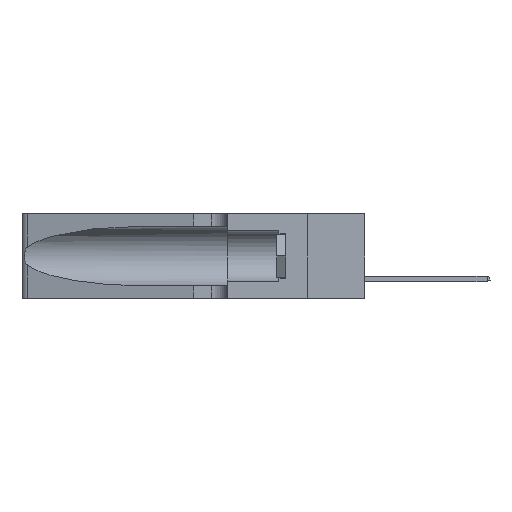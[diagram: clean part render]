
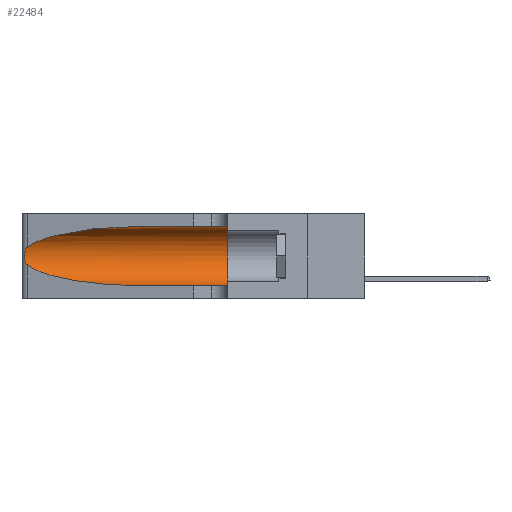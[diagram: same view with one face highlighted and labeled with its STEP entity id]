
A CAD part, left-side view. The second image highlights one B-rep face of the part: STEP entity #22484.
In plain terms, the highlighted cylindrical face has radius 3.308 mm (diameter 6.617 mm), a partial arc.
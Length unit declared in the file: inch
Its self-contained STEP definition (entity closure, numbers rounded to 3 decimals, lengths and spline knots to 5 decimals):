
#116 = DIRECTION ( 'NONE',  ( 0., -1., 0. ) ) ;
#454 = CARTESIAN_POINT ( 'NONE',  ( 0.18966, 0.96281, 0.05475 ) ) ;
#629 = CARTESIAN_POINT ( 'NONE',  ( 0.25787, 1.23484, 0.2124 ) ) ;
#763 = CARTESIAN_POINT ( 'NONE',  ( 0.25487, 1.22718, 0.14631 ) ) ;
#894 = CARTESIAN_POINT ( 'NONE',  ( 0.25555, 1.22994, 0.2215 ) ) ;
#1622 = EDGE_CURVE ( 'NONE', #23944, #12899, #24388, .T. ) ;
#1843 =( BOUNDED_CURVE ( )  B_SPLINE_CURVE ( 3, ( #36848, #27857, #454, #36561 ),
 .UNSPECIFIED., .F., .F. ) 
 B_SPLINE_CURVE_WITH_KNOTS ( ( 4, 4 ),
 ( 3.44316, 4.71239 ),
 .UNSPECIFIED. ) 
 CURVE ( )  GEOMETRIC_REPRESENTATION_ITEM ( )  RATIONAL_B_SPLINE_CURVE ( ( 1., 0.87, 0.87, 1. ) ) 
 REPRESENTATION_ITEM ( '' )  );
#3051 = LINE ( 'NONE', #29925, #14164 ) ;
#3424 = CARTESIAN_POINT ( 'NONE',  ( 0.26075, 1.23896, 0.19203 ) ) ;
#3725 = AXIS2_PLACEMENT_3D ( 'NONE', #30386, #30135, #12886 ) ;
#4051 = CARTESIAN_POINT ( 'NONE',  ( 0.1305, 0.35, 0.185 ) ) ;
#4172 = EDGE_CURVE ( 'NONE', #12899, #24948, #28204, .T. ) ;
#4389 = CARTESIAN_POINT ( 'NONE',  ( 0.25487, 1.22718, 0.14631 ) ) ;
#4609 = ORIENTED_EDGE ( 'NONE', *, *, #21694, .T. ) ;
#6536 = CARTESIAN_POINT ( 'NONE',  ( 0.1305, 0.35, 0.31525 ) ) ;
#8835 = CARTESIAN_POINT ( 'NONE',  ( 0.25856, 1.23593, 0.16098 ) ) ;
#10530 = CARTESIAN_POINT ( 'NONE',  ( 0.2373, 1.15595, 0.28018 ) ) ;
#11841 = ORIENTED_EDGE ( 'NONE', *, *, #25390, .T. ) ;
#12189 = CARTESIAN_POINT ( 'NONE',  ( 0.26018, 1.23835, 0.19895 ) ) ;
#12886 = DIRECTION ( 'NONE',  ( 0., 0., -1. ) ) ;
#12899 = VERTEX_POINT ( 'NONE', #6536 ) ;
#14164 = VECTOR ( 'NONE', #32774, 39.37008 ) ;
#15086 = CARTESIAN_POINT ( 'NONE',  ( 0.25789, 1.23486, 0.15765 ) ) ;
#15476 = DIRECTION ( 'NONE',  ( 0., 0., 1. ) ) ;
#16422 = CARTESIAN_POINT ( 'NONE',  ( 0.1305, 0.72297, 0.31525 ) ) ;
#16817 = VECTOR ( 'NONE', #116, 39.37008 ) ;
#16911 = AXIS2_PLACEMENT_3D ( 'NONE', #4051, #18142, #15476 ) ;
#16933 = EDGE_CURVE ( 'NONE', #23944, #20963, #36050, .T. ) ;
#17014 = CARTESIAN_POINT ( 'NONE',  ( 0.25487, 1.22718, 0.22369 ) ) ;
#17387 = EDGE_LOOP ( 'NONE', ( #27782, #11841, #26075, #4609, #18906, #19441 ) ) ;
#17864 = CARTESIAN_POINT ( 'NONE',  ( 0.25854, 1.2359, 0.20912 ) ) ;
#18142 = DIRECTION ( 'NONE',  ( 0., 1., 0. ) ) ;
#18906 = ORIENTED_EDGE ( 'NONE', *, *, #4172, .F. ) ;
#19441 = ORIENTED_EDGE ( 'NONE', *, *, #1622, .F. ) ;
#19479 = CARTESIAN_POINT ( 'NONE',  ( 0.25487, 1.22718, 0.22369 ) ) ;
#20963 = VERTEX_POINT ( 'NONE', #17014 ) ;
#21694 = EDGE_CURVE ( 'NONE', #27666, #24948, #3051, .T. ) ;
#21735 = VERTEX_POINT ( 'NONE', #4389 ) ;
#22058 = EDGE_CURVE ( 'NONE', #21735, #27666, #1843, .T. ) ;
#22484 = ADVANCED_FACE ( 'NONE', ( #23024 ), #25292, .F. ) ;
#22917 = CARTESIAN_POINT ( 'NONE',  ( 0.1305, 1.61858, 0.31525 ) ) ;
#23024 = FACE_OUTER_BOUND ( 'NONE', #17387, .T. ) ;
#23563 = CARTESIAN_POINT ( 'NONE',  ( 0.26017, 1.23833, 0.17102 ) ) ;
#23944 = VERTEX_POINT ( 'NONE', #32607 ) ;
#24388 = LINE ( 'NONE', #22917, #16817 ) ;
#24948 = VERTEX_POINT ( 'NONE', #26966 ) ;
#25292 = CYLINDRICAL_SURFACE ( 'NONE', #3725, 0.13025 ) ;
#25390 = EDGE_CURVE ( 'NONE', #20963, #21735, #28325, .T. ) ;
#26075 = ORIENTED_EDGE ( 'NONE', *, *, #22058, .T. ) ;
#26295 = CARTESIAN_POINT ( 'NONE',  ( 0.1305, 0.72297, 0.05475 ) ) ;
#26966 = CARTESIAN_POINT ( 'NONE',  ( 0.1305, 0.35, 0.05475 ) ) ;
#27666 = VERTEX_POINT ( 'NONE', #26295 ) ;
#27782 = ORIENTED_EDGE ( 'NONE', *, *, #16933, .T. ) ;
#27857 = CARTESIAN_POINT ( 'NONE',  ( 0.2373, 1.15595, 0.08982 ) ) ;
#28204 = CIRCLE ( 'NONE', #16911, 0.13025 ) ;
#28325 = B_SPLINE_CURVE_WITH_KNOTS ( 'NONE', 3,
 ( #32021, #894, #32163, #629, #17864, #12189, #3424, #29309, #23563, #8835, #15086, #29056, #28942, #763 ),
 .UNSPECIFIED., .F., .F.,
 ( 4, 2, 2, 2, 2, 2, 4 ),
 ( 0., 0.00027, 0.00053, 0.00107, 0.0016, 0.00187, 0.00214 ),
 .UNSPECIFIED. ) ;
#28942 = CARTESIAN_POINT ( 'NONE',  ( 0.25555, 1.22993, 0.14849 ) ) ;
#29056 = CARTESIAN_POINT ( 'NONE',  ( 0.25639, 1.23186, 0.15144 ) ) ;
#29309 = CARTESIAN_POINT ( 'NONE',  ( 0.26075, 1.23896, 0.178 ) ) ;
#29925 = CARTESIAN_POINT ( 'NONE',  ( 0.1305, 1.61858, 0.05475 ) ) ;
#30135 = DIRECTION ( 'NONE',  ( 0., -1., 0. ) ) ;
#30386 = CARTESIAN_POINT ( 'NONE',  ( 0.1305, 1.61858, 0.185 ) ) ;
#32021 = CARTESIAN_POINT ( 'NONE',  ( 0.25487, 1.22718, 0.22369 ) ) ;
#32163 = CARTESIAN_POINT ( 'NONE',  ( 0.25639, 1.23184, 0.21858 ) ) ;
#32607 = CARTESIAN_POINT ( 'NONE',  ( 0.1305, 0.72297, 0.31525 ) ) ;
#32774 = DIRECTION ( 'NONE',  ( 0., -1., 0. ) ) ;
#36050 =( BOUNDED_CURVE ( )  B_SPLINE_CURVE ( 3, ( #16422, #36210, #10530, #19479 ),
 .UNSPECIFIED., .F., .F. ) 
 B_SPLINE_CURVE_WITH_KNOTS ( ( 4, 4 ),
 ( 1.5708, 2.84003 ),
 .UNSPECIFIED. ) 
 CURVE ( )  GEOMETRIC_REPRESENTATION_ITEM ( )  RATIONAL_B_SPLINE_CURVE ( ( 1., 0.87, 0.87, 1. ) ) 
 REPRESENTATION_ITEM ( '' )  );
#36210 = CARTESIAN_POINT ( 'NONE',  ( 0.18966, 0.96281, 0.31525 ) ) ;
#36561 = CARTESIAN_POINT ( 'NONE',  ( 0.1305, 0.72297, 0.05475 ) ) ;
#36848 = CARTESIAN_POINT ( 'NONE',  ( 0.25487, 1.22718, 0.14631 ) ) ;
